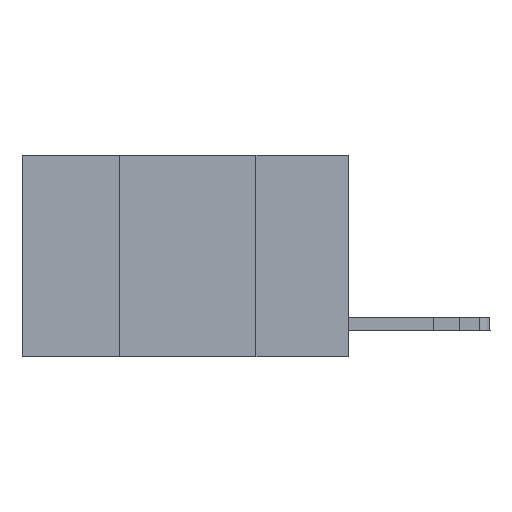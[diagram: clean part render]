
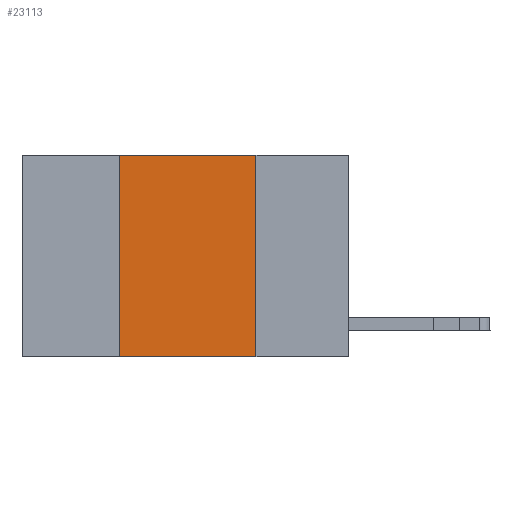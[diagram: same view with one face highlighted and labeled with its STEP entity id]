
A CAD part, left-side view. The second image highlights one B-rep face of the part: STEP entity #23113.
In plain terms, the highlighted planar face has unit normal (-1, 0, 0).
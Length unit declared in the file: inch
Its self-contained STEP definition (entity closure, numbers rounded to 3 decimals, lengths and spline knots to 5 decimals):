
#971 = VECTOR ( 'NONE', #12864, 39.37008 ) ;
#1547 = EDGE_CURVE ( 'NONE', #7335, #22639, #15764, .T. ) ;
#1802 = EDGE_CURVE ( 'NONE', #22639, #3979, #19153, .T. ) ;
#1867 = ORIENTED_EDGE ( 'NONE', *, *, #1547, .F. ) ;
#2786 = FACE_OUTER_BOUND ( 'NONE', #10480, .T. ) ;
#3979 = VERTEX_POINT ( 'NONE', #11685 ) ;
#4078 = CARTESIAN_POINT ( 'NONE',  ( 0., 0.17, 0. ) ) ;
#4954 = CARTESIAN_POINT ( 'NONE',  ( 0., 0.6, 0. ) ) ;
#4986 = PLANE ( 'NONE',  #16060 ) ;
#5210 = CARTESIAN_POINT ( 'NONE',  ( 0., 0.42, 0. ) ) ;
#5929 = LINE ( 'NONE', #20841, #7259 ) ;
#6389 = ORIENTED_EDGE ( 'NONE', *, *, #1802, .F. ) ;
#7259 = VECTOR ( 'NONE', #12489, 39.37008 ) ;
#7335 = VERTEX_POINT ( 'NONE', #5210 ) ;
#7474 = ORIENTED_EDGE ( 'NONE', *, *, #12859, .F. ) ;
#7739 = VERTEX_POINT ( 'NONE', #23838 ) ;
#8564 = DIRECTION ( 'NONE',  ( 0., -1., 0. ) ) ;
#8630 = VECTOR ( 'NONE', #20994, 39.37008 ) ;
#9174 = EDGE_CURVE ( 'NONE', #7739, #3979, #22577, .T. ) ;
#10159 = DIRECTION ( 'NONE',  ( 1., 0., 0. ) ) ;
#10480 = EDGE_LOOP ( 'NONE', ( #6389, #1867, #7474, #19900 ) ) ;
#10907 = CARTESIAN_POINT ( 'NONE',  ( 0., 0.6, -0.37 ) ) ;
#11685 = CARTESIAN_POINT ( 'NONE',  ( 0., 0.17, -0.37 ) ) ;
#11785 = CARTESIAN_POINT ( 'NONE',  ( 0., 0.17, 0. ) ) ;
#12489 = DIRECTION ( 'NONE',  ( 0., 0., 1. ) ) ;
#12859 = EDGE_CURVE ( 'NONE', #7739, #7335, #5929, .T. ) ;
#12864 = DIRECTION ( 'NONE',  ( 0., -1., 0. ) ) ;
#15764 = LINE ( 'NONE', #4954, #16455 ) ;
#16060 = AXIS2_PLACEMENT_3D ( 'NONE', #17513, #10159, #23205 ) ;
#16455 = VECTOR ( 'NONE', #8564, 39.37008 ) ;
#17513 = CARTESIAN_POINT ( 'NONE',  ( 0., 0.6, 0. ) ) ;
#19153 = LINE ( 'NONE', #11785, #8630 ) ;
#19900 = ORIENTED_EDGE ( 'NONE', *, *, #9174, .T. ) ;
#20841 = CARTESIAN_POINT ( 'NONE',  ( 0., 0.42, 0. ) ) ;
#20994 = DIRECTION ( 'NONE',  ( 0., 0., -1. ) ) ;
#22577 = LINE ( 'NONE', #10907, #971 ) ;
#22639 = VERTEX_POINT ( 'NONE', #4078 ) ;
#23113 = ADVANCED_FACE ( 'NONE', ( #2786 ), #4986, .F. ) ;
#23205 = DIRECTION ( 'NONE',  ( 0., 0., -1. ) ) ;
#23838 = CARTESIAN_POINT ( 'NONE',  ( 0., 0.42, -0.37 ) ) ;
